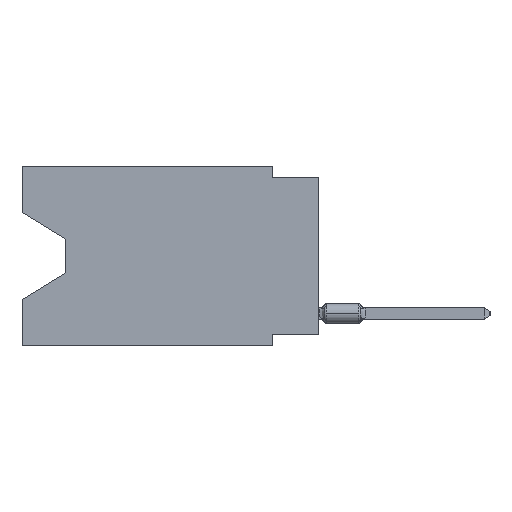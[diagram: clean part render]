
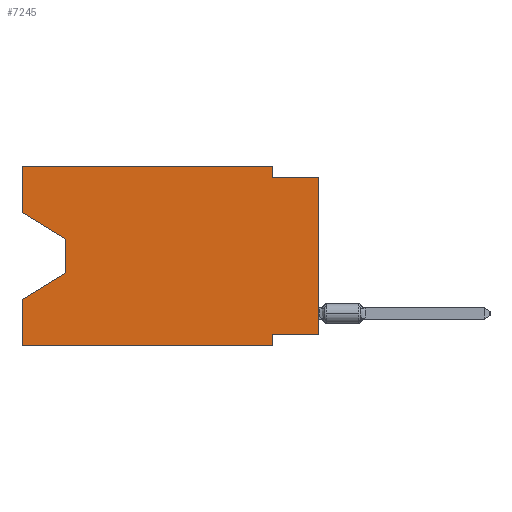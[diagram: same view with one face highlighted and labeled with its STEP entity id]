
A CAD part, left-side view. The second image highlights one B-rep face of the part: STEP entity #7245.
In plain terms, the highlighted planar face has unit normal (-1, 0, 0).
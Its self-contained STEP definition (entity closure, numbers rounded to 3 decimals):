
#1259 = ORIENTED_EDGE ( 'NONE', *, *, #17842, .F. ) ;
#1465 = EDGE_CURVE ( 'NONE', #25862, #21515, #23876, .T. ) ;
#1480 = ORIENTED_EDGE ( 'NONE', *, *, #9246, .F. ) ;
#1496 = VECTOR ( 'NONE', #29755, 1000. ) ;
#1536 = FACE_OUTER_BOUND ( 'NONE', #14994, .T. ) ;
#1759 = VERTEX_POINT ( 'NONE', #15055 ) ;
#1981 = ORIENTED_EDGE ( 'NONE', *, *, #31053, .F. ) ;
#2026 = VERTEX_POINT ( 'NONE', #19922 ) ;
#2151 = VERTEX_POINT ( 'NONE', #5213 ) ;
#2383 = VECTOR ( 'NONE', #11967, 1000. ) ;
#2545 = VERTEX_POINT ( 'NONE', #25427 ) ;
#3026 = CARTESIAN_POINT ( 'NONE',  ( 0., 16.383, -9.906 ) ) ;
#3028 = VERTEX_POINT ( 'NONE', #10201 ) ;
#3278 = EDGE_CURVE ( 'NONE', #10544, #1759, #20394, .T. ) ;
#4385 = EDGE_CURVE ( 'NONE', #2151, #18381, #8252, .T. ) ;
#4514 = ORIENTED_EDGE ( 'NONE', *, *, #17640, .T. ) ;
#4867 = VERTEX_POINT ( 'NONE', #22227 ) ;
#5213 = CARTESIAN_POINT ( 'NONE',  ( 0., 16.383, -9.906 ) ) ;
#5462 = CARTESIAN_POINT ( 'NONE',  ( 0., 16.383, 0. ) ) ;
#5537 = VERTEX_POINT ( 'NONE', #26060 ) ;
#5649 = EDGE_CURVE ( 'NONE', #5537, #3028, #9309, .T. ) ;
#5742 = DIRECTION ( 'NONE',  ( 0., 0., -1. ) ) ;
#6437 = VERTEX_POINT ( 'NONE', #23926 ) ;
#6577 = DIRECTION ( 'NONE',  ( 0., 0., -1. ) ) ;
#6855 = CARTESIAN_POINT ( 'NONE',  ( 0., 0., -9.271 ) ) ;
#7245 = ADVANCED_FACE ( 'NONE', ( #1536 ), #24969, .F. ) ;
#7628 = CARTESIAN_POINT ( 'NONE',  ( 0., 0., -0.635 ) ) ;
#7981 = VECTOR ( 'NONE', #5742, 1000. ) ;
#8252 = LINE ( 'NONE', #3026, #20262 ) ;
#8368 = CARTESIAN_POINT ( 'NONE',  ( 0., 2.54, -9.906 ) ) ;
#8582 = ORIENTED_EDGE ( 'NONE', *, *, #24716, .F. ) ;
#9246 = EDGE_CURVE ( 'NONE', #2026, #18381, #19583, .T. ) ;
#9309 = LINE ( 'NONE', #11531, #16969 ) ;
#9330 = ORIENTED_EDGE ( 'NONE', *, *, #4385, .T. ) ;
#9553 = CARTESIAN_POINT ( 'NONE',  ( 0., 0., 0. ) ) ;
#10135 = DIRECTION ( 'NONE',  ( 0., 0., 1. ) ) ;
#10201 = CARTESIAN_POINT ( 'NONE',  ( 0., 16.383, -7.36 ) ) ;
#10224 = ORIENTED_EDGE ( 'NONE', *, *, #3278, .T. ) ;
#10269 = DIRECTION ( 'NONE',  ( 0., -1., 0. ) ) ;
#10544 = VERTEX_POINT ( 'NONE', #20800 ) ;
#10881 = CARTESIAN_POINT ( 'NONE',  ( 0., 16.383, -2.546 ) ) ;
#11531 = CARTESIAN_POINT ( 'NONE',  ( 0., 13.97, -5.893 ) ) ;
#11814 = CARTESIAN_POINT ( 'NONE',  ( 0., 2.54, -9.906 ) ) ;
#11967 = DIRECTION ( 'NONE',  ( 0., 0., -1. ) ) ;
#12985 = CARTESIAN_POINT ( 'NONE',  ( 0., 16.383, 0. ) ) ;
#13701 = EDGE_CURVE ( 'NONE', #10544, #2026, #13999, .T. ) ;
#13999 = LINE ( 'NONE', #6855, #18730 ) ;
#14293 = EDGE_CURVE ( 'NONE', #25862, #6437, #18840, .T. ) ;
#14606 = ORIENTED_EDGE ( 'NONE', *, *, #14293, .T. ) ;
#14994 = EDGE_LOOP ( 'NONE', ( #14606, #4514, #31123, #17737, #9330, #1480, #15289, #10224, #8582, #1981, #1259, #26675 ) ) ;
#15055 = CARTESIAN_POINT ( 'NONE',  ( 0., 0., -0.635 ) ) ;
#15168 = LINE ( 'NONE', #12985, #19853 ) ;
#15289 = ORIENTED_EDGE ( 'NONE', *, *, #13701, .F. ) ;
#15496 = CARTESIAN_POINT ( 'NONE',  ( 0., 16.383, 0. ) ) ;
#16740 = DIRECTION ( 'NONE',  ( 1., 0., 0. ) ) ;
#16969 = VECTOR ( 'NONE', #19155, 1000. ) ;
#17640 = EDGE_CURVE ( 'NONE', #6437, #5537, #18591, .T. ) ;
#17737 = ORIENTED_EDGE ( 'NONE', *, *, #26350, .F. ) ;
#17842 = EDGE_CURVE ( 'NONE', #21515, #2545, #15168, .T. ) ;
#18381 = VERTEX_POINT ( 'NONE', #8368 ) ;
#18591 = LINE ( 'NONE', #28869, #7981 ) ;
#18730 = VECTOR ( 'NONE', #27450, 1000. ) ;
#18840 = LINE ( 'NONE', #10881, #21743 ) ;
#19155 = DIRECTION ( 'NONE',  ( 0., 0.855, -0.519 ) ) ;
#19583 = LINE ( 'NONE', #11814, #2383 ) ;
#19853 = VECTOR ( 'NONE', #10269, 1000. ) ;
#19922 = CARTESIAN_POINT ( 'NONE',  ( 0., 2.54, -9.271 ) ) ;
#20099 = LINE ( 'NONE', #33068, #31222 ) ;
#20262 = VECTOR ( 'NONE', #26145, 1000. ) ;
#20394 = LINE ( 'NONE', #9553, #26959 ) ;
#20800 = CARTESIAN_POINT ( 'NONE',  ( 0., 0., -9.271 ) ) ;
#21515 = VERTEX_POINT ( 'NONE', #15496 ) ;
#21743 = VECTOR ( 'NONE', #31473, 1000. ) ;
#22227 = CARTESIAN_POINT ( 'NONE',  ( 0., 2.54, -0.635 ) ) ;
#22298 = CARTESIAN_POINT ( 'NONE',  ( 0., 16.383, 0. ) ) ;
#23086 = DIRECTION ( 'NONE',  ( 0., 0., 1. ) ) ;
#23876 = LINE ( 'NONE', #5462, #28983 ) ;
#23891 = CARTESIAN_POINT ( 'NONE',  ( 0., 2.54, 0. ) ) ;
#23926 = CARTESIAN_POINT ( 'NONE',  ( 0., 13.97, -4.013 ) ) ;
#24716 = EDGE_CURVE ( 'NONE', #4867, #1759, #30762, .T. ) ;
#24969 = PLANE ( 'NONE',  #26541 ) ;
#25427 = CARTESIAN_POINT ( 'NONE',  ( 0., 2.54, 0. ) ) ;
#25862 = VERTEX_POINT ( 'NONE', #28223 ) ;
#26060 = CARTESIAN_POINT ( 'NONE',  ( 0., 13.97, -5.893 ) ) ;
#26145 = DIRECTION ( 'NONE',  ( 0., -1., 0. ) ) ;
#26304 = VECTOR ( 'NONE', #28214, 1000. ) ;
#26350 = EDGE_CURVE ( 'NONE', #2151, #3028, #20099, .T. ) ;
#26541 = AXIS2_PLACEMENT_3D ( 'NONE', #22298, #16740, #6577 ) ;
#26675 = ORIENTED_EDGE ( 'NONE', *, *, #1465, .F. ) ;
#26959 = VECTOR ( 'NONE', #23086, 1000. ) ;
#27450 = DIRECTION ( 'NONE',  ( 0., 1., 0. ) ) ;
#28214 = DIRECTION ( 'NONE',  ( 0., -1., 0. ) ) ;
#28223 = CARTESIAN_POINT ( 'NONE',  ( 0., 16.383, -2.546 ) ) ;
#28869 = CARTESIAN_POINT ( 'NONE',  ( 0., 13.97, -4.013 ) ) ;
#28983 = VECTOR ( 'NONE', #31305, 1000. ) ;
#29755 = DIRECTION ( 'NONE',  ( 0., 0., -1. ) ) ;
#30762 = LINE ( 'NONE', #7628, #26304 ) ;
#31053 = EDGE_CURVE ( 'NONE', #2545, #4867, #31652, .T. ) ;
#31123 = ORIENTED_EDGE ( 'NONE', *, *, #5649, .T. ) ;
#31222 = VECTOR ( 'NONE', #10135, 1000. ) ;
#31305 = DIRECTION ( 'NONE',  ( 0., 0., 1. ) ) ;
#31473 = DIRECTION ( 'NONE',  ( 0., -0.855, -0.519 ) ) ;
#31652 = LINE ( 'NONE', #23891, #1496 ) ;
#33068 = CARTESIAN_POINT ( 'NONE',  ( 0., 16.383, 0. ) ) ;
